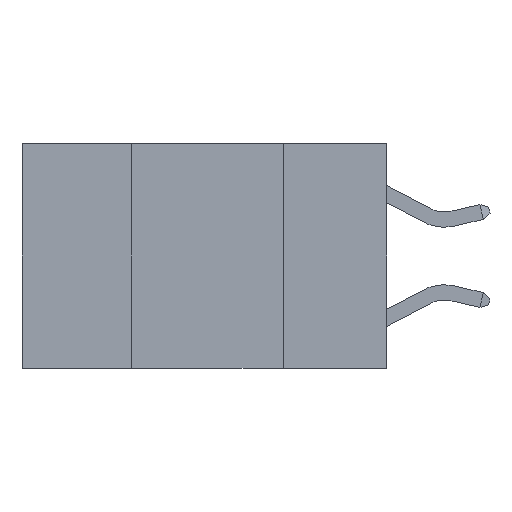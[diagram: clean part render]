
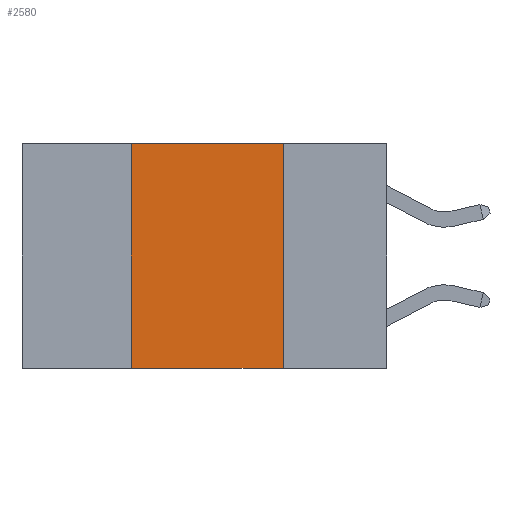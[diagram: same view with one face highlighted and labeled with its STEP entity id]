
A CAD part, left-side view. The second image highlights one B-rep face of the part: STEP entity #2580.
In plain terms, the highlighted planar face has unit normal (-1, 0, 0).
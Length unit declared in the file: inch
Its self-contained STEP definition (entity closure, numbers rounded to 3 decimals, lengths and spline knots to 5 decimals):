
#497 = LINE ( 'NONE', #8856, #8273 ) ;
#748 = CARTESIAN_POINT ( 'NONE',  ( 0., 0.17, 0. ) ) ;
#909 = ORIENTED_EDGE ( 'NONE', *, *, #5476, .T. ) ;
#1538 = DIRECTION ( 'NONE',  ( 0., 0., -1. ) ) ;
#1752 = DIRECTION ( 'NONE',  ( 0., -1., 0. ) ) ;
#2485 = ORIENTED_EDGE ( 'NONE', *, *, #6496, .F. ) ;
#2496 = ORIENTED_EDGE ( 'NONE', *, *, #2639, .F. ) ;
#2580 = ADVANCED_FACE ( 'NONE', ( #7295 ), #6484, .F. ) ;
#2639 = EDGE_CURVE ( 'NONE', #5716, #6028, #8713, .T. ) ;
#3011 = CARTESIAN_POINT ( 'NONE',  ( 0., 0.42, -0.37 ) ) ;
#3130 = VERTEX_POINT ( 'NONE', #3011 ) ;
#3564 = CARTESIAN_POINT ( 'NONE',  ( 0., 0.42, 0. ) ) ;
#3785 = ORIENTED_EDGE ( 'NONE', *, *, #6589, .F. ) ;
#5267 = DIRECTION ( 'NONE',  ( 0., 0., 1. ) ) ;
#5476 = EDGE_CURVE ( 'NONE', #3130, #8493, #8358, .T. ) ;
#5526 = CARTESIAN_POINT ( 'NONE',  ( 0., 0.6, -0.37 ) ) ;
#5716 = VERTEX_POINT ( 'NONE', #3564 ) ;
#5738 = AXIS2_PLACEMENT_3D ( 'NONE', #6446, #6443, #6435 ) ;
#6016 = EDGE_LOOP ( 'NONE', ( #3785, #2496, #2485, #909 ) ) ;
#6028 = VERTEX_POINT ( 'NONE', #7589 ) ;
#6076 = DIRECTION ( 'NONE',  ( 0., -1., 0. ) ) ;
#6162 = CARTESIAN_POINT ( 'NONE',  ( 0., 0.6, 0. ) ) ;
#6435 = DIRECTION ( 'NONE',  ( 0., 0., -1. ) ) ;
#6443 = DIRECTION ( 'NONE',  ( 1., 0., 0. ) ) ;
#6446 = CARTESIAN_POINT ( 'NONE',  ( 0., 0.6, 0. ) ) ;
#6452 = VECTOR ( 'NONE', #1752, 39.37008 ) ;
#6484 = PLANE ( 'NONE',  #5738 ) ;
#6496 = EDGE_CURVE ( 'NONE', #3130, #5716, #497, .T. ) ;
#6589 = EDGE_CURVE ( 'NONE', #6028, #8493, #7812, .T. ) ;
#6619 = VECTOR ( 'NONE', #6076, 39.37008 ) ;
#7070 = CARTESIAN_POINT ( 'NONE',  ( 0., 0.17, -0.37 ) ) ;
#7295 = FACE_OUTER_BOUND ( 'NONE', #6016, .T. ) ;
#7589 = CARTESIAN_POINT ( 'NONE',  ( 0., 0.17, 0. ) ) ;
#7598 = VECTOR ( 'NONE', #1538, 39.37008 ) ;
#7812 = LINE ( 'NONE', #748, #7598 ) ;
#8273 = VECTOR ( 'NONE', #5267, 39.37008 ) ;
#8358 = LINE ( 'NONE', #5526, #6452 ) ;
#8493 = VERTEX_POINT ( 'NONE', #7070 ) ;
#8713 = LINE ( 'NONE', #6162, #6619 ) ;
#8856 = CARTESIAN_POINT ( 'NONE',  ( 0., 0.42, 0. ) ) ;
